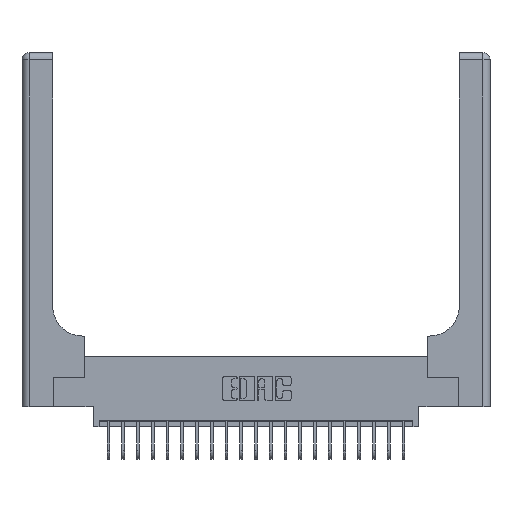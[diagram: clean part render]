
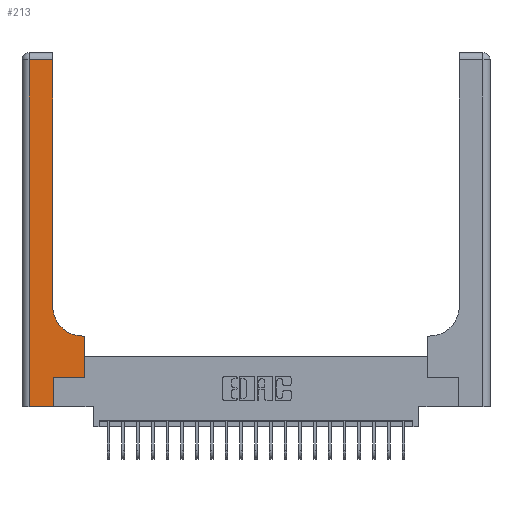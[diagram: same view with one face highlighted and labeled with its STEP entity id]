
A CAD part, top view. The second image highlights one B-rep face of the part: STEP entity #213.
In plain terms, the highlighted planar face has unit normal (0, 0, 1).
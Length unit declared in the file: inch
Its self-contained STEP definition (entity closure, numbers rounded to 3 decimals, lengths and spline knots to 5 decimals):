
#213 = ADVANCED_FACE ( 'NONE', ( #3478 ), #6388, .F. ) ;
#400 = AXIS2_PLACEMENT_3D ( 'NONE', #11916, #6303, #13752 ) ;
#436 = ORIENTED_EDGE ( 'NONE', *, *, #15059, .T. ) ;
#688 = VERTEX_POINT ( 'NONE', #714 ) ;
#714 = CARTESIAN_POINT ( 'NONE',  ( 0.26, 0.85, 0.37 ) ) ;
#811 = VECTOR ( 'NONE', #6738, 39.37008 ) ;
#1061 = DIRECTION ( 'NONE',  ( -1., 0., 0. ) ) ;
#1550 = LINE ( 'NONE', #17449, #16704 ) ;
#1871 = AXIS2_PLACEMENT_3D ( 'NONE', #3269, #8746, #5121 ) ;
#1875 = VECTOR ( 'NONE', #17492, 39.37008 ) ;
#2167 = EDGE_LOOP ( 'NONE', ( #10091, #16748, #17483, #13227, #436, #21416, #18122, #4837, #10529 ) ) ;
#2780 = EDGE_CURVE ( 'NONE', #16751, #6546, #17962, .T. ) ;
#3192 = EDGE_CURVE ( 'NONE', #13804, #10920, #4772, .T. ) ;
#3269 = CARTESIAN_POINT ( 'NONE',  ( 0.51, 0.85, 0.37 ) ) ;
#3412 = CARTESIAN_POINT ( 'NONE',  ( 0.06, 0., 0.37 ) ) ;
#3478 = FACE_OUTER_BOUND ( 'NONE', #2167, .T. ) ;
#3890 = CARTESIAN_POINT ( 'NONE',  ( 0.265, 0., 0.37 ) ) ;
#3985 = CARTESIAN_POINT ( 'NONE',  ( 0., 2.94, 0.37 ) ) ;
#4102 = VECTOR ( 'NONE', #16295, 39.37008 ) ;
#4541 = DIRECTION ( 'NONE',  ( -1., 0., 0. ) ) ;
#4543 = EDGE_CURVE ( 'NONE', #13205, #13804, #23310, .T. ) ;
#4772 = LINE ( 'NONE', #5082, #18227 ) ;
#4837 = ORIENTED_EDGE ( 'NONE', *, *, #10142, .T. ) ;
#5082 = CARTESIAN_POINT ( 'NONE',  ( 0., 0., 0.37 ) ) ;
#5121 = DIRECTION ( 'NONE',  ( 1., 0., 0. ) ) ;
#6303 = DIRECTION ( 'NONE',  ( 0., 0., -1. ) ) ;
#6388 = PLANE ( 'NONE',  #400 ) ;
#6546 = VERTEX_POINT ( 'NONE', #9052 ) ;
#6738 = DIRECTION ( 'NONE',  ( 1., 0., 0. ) ) ;
#7430 = CARTESIAN_POINT ( 'NONE',  ( 0.528, 0.6, 0.37 ) ) ;
#7461 = DIRECTION ( 'NONE',  ( 0., 1., 0. ) ) ;
#7699 = CARTESIAN_POINT ( 'NONE',  ( 0.26, 3., 0.37 ) ) ;
#7799 = VECTOR ( 'NONE', #4541, 39.37008 ) ;
#8585 = EDGE_CURVE ( 'NONE', #688, #16555, #20700, .T. ) ;
#8746 = DIRECTION ( 'NONE',  ( 0., 0., -1. ) ) ;
#8782 = DIRECTION ( 'NONE',  ( 1., 0., 0. ) ) ;
#9052 = CARTESIAN_POINT ( 'NONE',  ( 0.528, 0.25, 0.37 ) ) ;
#9885 = CARTESIAN_POINT ( 'NONE',  ( 0.265, 0., 0.37 ) ) ;
#10091 = ORIENTED_EDGE ( 'NONE', *, *, #8585, .T. ) ;
#10142 = EDGE_CURVE ( 'NONE', #18289, #19745, #1550, .T. ) ;
#10446 = EDGE_CURVE ( 'NONE', #6546, #18289, #15264, .T. ) ;
#10529 = ORIENTED_EDGE ( 'NONE', *, *, #22654, .T. ) ;
#10920 = VERTEX_POINT ( 'NONE', #3890 ) ;
#11123 = VECTOR ( 'NONE', #22493, 39.37008 ) ;
#11894 = EDGE_CURVE ( 'NONE', #16555, #13205, #17519, .T. ) ;
#11916 = CARTESIAN_POINT ( 'NONE',  ( 0., 3., 0.37 ) ) ;
#13205 = VERTEX_POINT ( 'NONE', #22882 ) ;
#13227 = ORIENTED_EDGE ( 'NONE', *, *, #3192, .T. ) ;
#13752 = DIRECTION ( 'NONE',  ( -1., 0., 0. ) ) ;
#13767 = CARTESIAN_POINT ( 'NONE',  ( 0.51, 0.6, 0.37 ) ) ;
#13804 = VERTEX_POINT ( 'NONE', #3412 ) ;
#14250 = LINE ( 'NONE', #9885, #11123 ) ;
#15059 = EDGE_CURVE ( 'NONE', #10920, #16751, #14250, .T. ) ;
#15264 = LINE ( 'NONE', #21685, #4102 ) ;
#15521 = CARTESIAN_POINT ( 'NONE',  ( 0.265, 0.25, 0.37 ) ) ;
#15569 = CARTESIAN_POINT ( 'NONE',  ( 0.06, 3., 0.37 ) ) ;
#15736 = CIRCLE ( 'NONE', #1871, 0.25 ) ;
#16295 = DIRECTION ( 'NONE',  ( 0., 1., 0. ) ) ;
#16555 = VERTEX_POINT ( 'NONE', #22264 ) ;
#16704 = VECTOR ( 'NONE', #1061, 39.37008 ) ;
#16748 = ORIENTED_EDGE ( 'NONE', *, *, #11894, .T. ) ;
#16751 = VERTEX_POINT ( 'NONE', #15521 ) ;
#16932 = VECTOR ( 'NONE', #7461, 39.37008 ) ;
#17449 = CARTESIAN_POINT ( 'NONE',  ( 0.26, 0.6, 0.37 ) ) ;
#17483 = ORIENTED_EDGE ( 'NONE', *, *, #4543, .T. ) ;
#17492 = DIRECTION ( 'NONE',  ( 0., -1., 0. ) ) ;
#17519 = LINE ( 'NONE', #3985, #7799 ) ;
#17962 = LINE ( 'NONE', #23191, #811 ) ;
#18122 = ORIENTED_EDGE ( 'NONE', *, *, #10446, .T. ) ;
#18227 = VECTOR ( 'NONE', #8782, 39.37008 ) ;
#18289 = VERTEX_POINT ( 'NONE', #7430 ) ;
#19745 = VERTEX_POINT ( 'NONE', #13767 ) ;
#20700 = LINE ( 'NONE', #7699, #16932 ) ;
#21416 = ORIENTED_EDGE ( 'NONE', *, *, #2780, .T. ) ;
#21685 = CARTESIAN_POINT ( 'NONE',  ( 0.528, 0.25, 0.37 ) ) ;
#22264 = CARTESIAN_POINT ( 'NONE',  ( 0.26, 2.94, 0.37 ) ) ;
#22493 = DIRECTION ( 'NONE',  ( 0., 1., 0. ) ) ;
#22654 = EDGE_CURVE ( 'NONE', #19745, #688, #15736, .T. ) ;
#22882 = CARTESIAN_POINT ( 'NONE',  ( 0.06, 2.94, 0.37 ) ) ;
#23191 = CARTESIAN_POINT ( 'NONE',  ( 0.265, 0.25, 0.37 ) ) ;
#23310 = LINE ( 'NONE', #15569, #1875 ) ;
